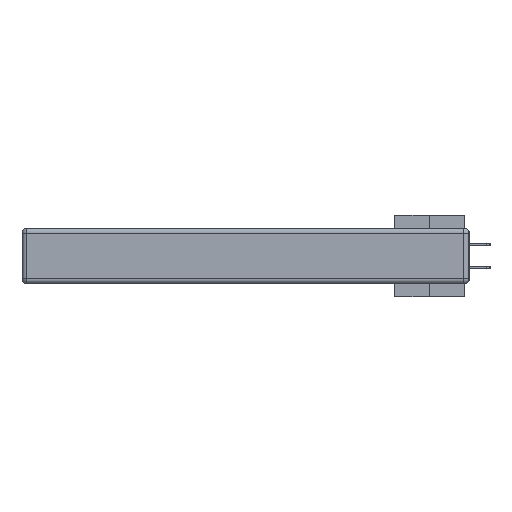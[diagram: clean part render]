
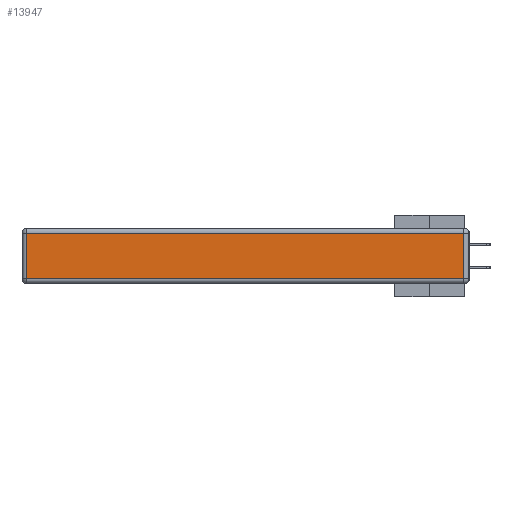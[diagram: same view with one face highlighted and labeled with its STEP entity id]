
A CAD part, left-side view. The second image highlights one B-rep face of the part: STEP entity #13947.
In plain terms, the highlighted planar face has unit normal (-1, 0, 0).
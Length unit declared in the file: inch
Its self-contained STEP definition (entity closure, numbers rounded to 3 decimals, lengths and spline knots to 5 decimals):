
#536 = LINE ( 'NONE', #27070, #30239 ) ;
#1448 = AXIS2_PLACEMENT_3D ( 'NONE', #11994, #29689, #35960 ) ;
#1818 = VERTEX_POINT ( 'NONE', #18689 ) ;
#1867 = VECTOR ( 'NONE', #9811, 39.37008 ) ;
#3796 = VERTEX_POINT ( 'NONE', #13925 ) ;
#7806 = EDGE_CURVE ( 'NONE', #33845, #20903, #11067, .T. ) ;
#9257 = CARTESIAN_POINT ( 'NONE',  ( 0., 2.72, -0.03 ) ) ;
#9420 = CARTESIAN_POINT ( 'NONE',  ( 0., 2.75, -0.03 ) ) ;
#9811 = DIRECTION ( 'NONE',  ( 0., 1., 0. ) ) ;
#11067 = LINE ( 'NONE', #24352, #11512 ) ;
#11512 = VECTOR ( 'NONE', #24232, 39.37008 ) ;
#11606 = DIRECTION ( 'NONE',  ( 0., 0., 1. ) ) ;
#11994 = CARTESIAN_POINT ( 'NONE',  ( 0., 0., -0.343 ) ) ;
#12434 = EDGE_CURVE ( 'NONE', #20903, #1818, #536, .T. ) ;
#13098 = EDGE_CURVE ( 'NONE', #1818, #3796, #31489, .T. ) ;
#13884 = ORIENTED_EDGE ( 'NONE', *, *, #13098, .T. ) ;
#13925 = CARTESIAN_POINT ( 'NONE',  ( 0., 0.03, -0.03 ) ) ;
#13947 = ADVANCED_FACE ( 'NONE', ( #19863 ), #23722, .T. ) ;
#18475 = ORIENTED_EDGE ( 'NONE', *, *, #7806, .T. ) ;
#18689 = CARTESIAN_POINT ( 'NONE',  ( 0., 0.03, -0.313 ) ) ;
#19460 = LINE ( 'NONE', #9420, #1867 ) ;
#19863 = FACE_OUTER_BOUND ( 'NONE', #36508, .T. ) ;
#20903 = VERTEX_POINT ( 'NONE', #26935 ) ;
#23249 = EDGE_CURVE ( 'NONE', #3796, #33845, #19460, .T. ) ;
#23592 = CARTESIAN_POINT ( 'NONE',  ( 0., 0.03, -0.343 ) ) ;
#23722 = PLANE ( 'NONE',  #1448 ) ;
#24232 = DIRECTION ( 'NONE',  ( 0., 0., -1. ) ) ;
#24352 = CARTESIAN_POINT ( 'NONE',  ( 0., 2.72, -0.343 ) ) ;
#26935 = CARTESIAN_POINT ( 'NONE',  ( 0., 2.72, -0.313 ) ) ;
#27070 = CARTESIAN_POINT ( 'NONE',  ( 0., 0., -0.313 ) ) ;
#27324 = DIRECTION ( 'NONE',  ( 0., -1., 0. ) ) ;
#29689 = DIRECTION ( 'NONE',  ( -1., 0., 0. ) ) ;
#30239 = VECTOR ( 'NONE', #27324, 39.37008 ) ;
#31489 = LINE ( 'NONE', #23592, #38503 ) ;
#33845 = VERTEX_POINT ( 'NONE', #9257 ) ;
#35960 = DIRECTION ( 'NONE',  ( 0., 0., 1. ) ) ;
#36508 = EDGE_LOOP ( 'NONE', ( #36679, #13884, #36579, #18475 ) ) ;
#36579 = ORIENTED_EDGE ( 'NONE', *, *, #23249, .T. ) ;
#36679 = ORIENTED_EDGE ( 'NONE', *, *, #12434, .T. ) ;
#38503 = VECTOR ( 'NONE', #11606, 39.37008 ) ;
